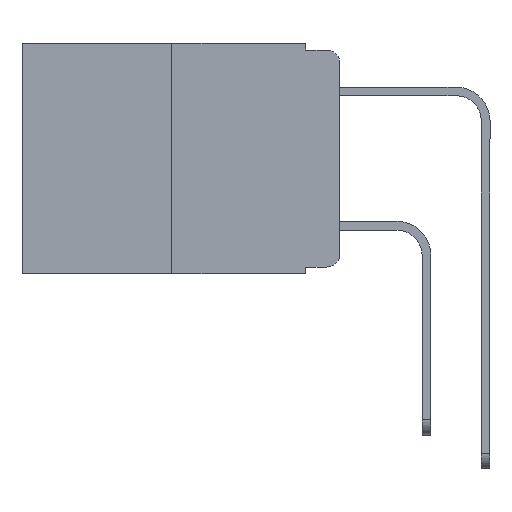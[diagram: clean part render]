
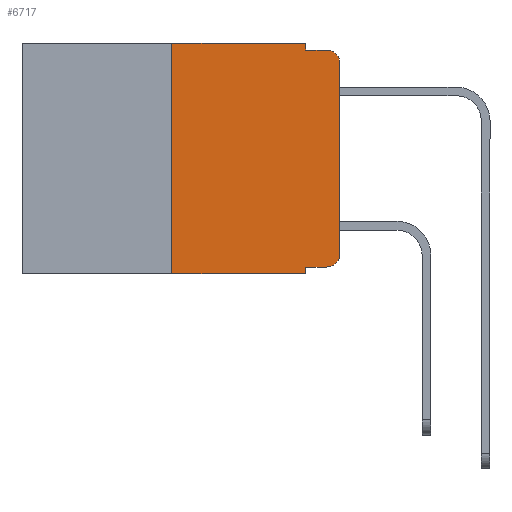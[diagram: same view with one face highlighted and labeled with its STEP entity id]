
A CAD part, left-side view. The second image highlights one B-rep face of the part: STEP entity #6717.
In plain terms, the highlighted planar face has unit normal (-1, 0, 0).
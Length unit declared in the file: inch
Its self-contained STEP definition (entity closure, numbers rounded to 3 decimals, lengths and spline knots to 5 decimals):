
#454 = LINE ( 'NONE', #2485, #11881 ) ;
#506 = DIRECTION ( 'NONE',  ( 0., 0., -1. ) ) ;
#592 = CARTESIAN_POINT ( 'NONE',  ( 0., 0.051, -0.333 ) ) ;
#717 = CIRCLE ( 'NONE', #2835, 0.02 ) ;
#940 = EDGE_CURVE ( 'NONE', #14109, #8351, #7957, .T. ) ;
#1337 = CARTESIAN_POINT ( 'NONE',  ( 0., 0.25, 0. ) ) ;
#1345 = DIRECTION ( 'NONE',  ( 0., 0., 1. ) ) ;
#1373 = VECTOR ( 'NONE', #1345, 39.37008 ) ;
#1735 = VECTOR ( 'NONE', #13034, 39.37008 ) ;
#1844 = EDGE_CURVE ( 'NONE', #14109, #13700, #3982, .T. ) ;
#1927 = VERTEX_POINT ( 'NONE', #11083 ) ;
#2132 = ORIENTED_EDGE ( 'NONE', *, *, #14642, .T. ) ;
#2195 = EDGE_LOOP ( 'NONE', ( #5066, #6469, #6988, #11671, #12996, #7486, #2898, #10226, #9751, #2132 ) ) ;
#2341 = CIRCLE ( 'NONE', #6979, 0.02 ) ;
#2485 = CARTESIAN_POINT ( 'NONE',  ( 0., 0.473, -0.343 ) ) ;
#2699 = EDGE_CURVE ( 'NONE', #11768, #9002, #4660, .T. ) ;
#2835 = AXIS2_PLACEMENT_3D ( 'NONE', #13978, #7622, #506 ) ;
#2898 = ORIENTED_EDGE ( 'NONE', *, *, #3746, .T. ) ;
#3273 = DIRECTION ( 'NONE',  ( -1., 0., 0. ) ) ;
#3292 = CARTESIAN_POINT ( 'NONE',  ( 0., 0.051, -0.01 ) ) ;
#3385 = DIRECTION ( 'NONE',  ( 0., -1., 0. ) ) ;
#3554 = EDGE_CURVE ( 'NONE', #8930, #12982, #8603, .T. ) ;
#3745 = CARTESIAN_POINT ( 'NONE',  ( 0., 0.473, 0. ) ) ;
#3746 = EDGE_CURVE ( 'NONE', #11768, #13700, #454, .T. ) ;
#3982 = LINE ( 'NONE', #14052, #11631 ) ;
#4300 = EDGE_CURVE ( 'NONE', #12982, #7825, #10400, .T. ) ;
#4369 = CARTESIAN_POINT ( 'NONE',  ( 0., 0.051, 0. ) ) ;
#4660 = LINE ( 'NONE', #14540, #1373 ) ;
#5062 = EDGE_CURVE ( 'NONE', #1927, #7825, #2341, .T. ) ;
#5066 = ORIENTED_EDGE ( 'NONE', *, *, #6547, .T. ) ;
#5121 = AXIS2_PLACEMENT_3D ( 'NONE', #10971, #6692, #14125 ) ;
#5256 = CARTESIAN_POINT ( 'NONE',  ( 0., 0.25, -0.343 ) ) ;
#5494 = DIRECTION ( 'NONE',  ( 0., 0., -1. ) ) ;
#5903 = CARTESIAN_POINT ( 'NONE',  ( 0., 0.051, 0. ) ) ;
#6469 = ORIENTED_EDGE ( 'NONE', *, *, #5062, .T. ) ;
#6547 = EDGE_CURVE ( 'NONE', #11022, #1927, #8547, .T. ) ;
#6692 = DIRECTION ( 'NONE',  ( 1., 0., 0. ) ) ;
#6717 = ADVANCED_FACE ( 'NONE', ( #9396 ), #13075, .F. ) ;
#6979 = AXIS2_PLACEMENT_3D ( 'NONE', #9922, #3273, #10957 ) ;
#6988 = ORIENTED_EDGE ( 'NONE', *, *, #4300, .F. ) ;
#7024 = VECTOR ( 'NONE', #7108, 39.37008 ) ;
#7108 = DIRECTION ( 'NONE',  ( 0., -1., 0. ) ) ;
#7441 = CARTESIAN_POINT ( 'NONE',  ( 0., 0., 0. ) ) ;
#7466 = CARTESIAN_POINT ( 'NONE',  ( 0., 0., -0.313 ) ) ;
#7486 = ORIENTED_EDGE ( 'NONE', *, *, #2699, .F. ) ;
#7622 = DIRECTION ( 'NONE',  ( -1., 0., 0. ) ) ;
#7825 = VERTEX_POINT ( 'NONE', #11664 ) ;
#7957 = LINE ( 'NONE', #13167, #12925 ) ;
#8193 = DIRECTION ( 'NONE',  ( 0., -1., 0. ) ) ;
#8351 = VERTEX_POINT ( 'NONE', #10460 ) ;
#8547 = LINE ( 'NONE', #7441, #11015 ) ;
#8603 = LINE ( 'NONE', #4369, #11388 ) ;
#8622 = DIRECTION ( 'NONE',  ( 0., 0., 1. ) ) ;
#8930 = VERTEX_POINT ( 'NONE', #5903 ) ;
#9002 = VERTEX_POINT ( 'NONE', #1337 ) ;
#9396 = FACE_OUTER_BOUND ( 'NONE', #2195, .T. ) ;
#9751 = ORIENTED_EDGE ( 'NONE', *, *, #940, .T. ) ;
#9884 = CARTESIAN_POINT ( 'NONE',  ( 0., 0.051, -0.01 ) ) ;
#9922 = CARTESIAN_POINT ( 'NONE',  ( 0., 0.02, -0.03 ) ) ;
#10226 = ORIENTED_EDGE ( 'NONE', *, *, #1844, .F. ) ;
#10400 = LINE ( 'NONE', #3292, #1735 ) ;
#10460 = CARTESIAN_POINT ( 'NONE',  ( 0., 0.02, -0.333 ) ) ;
#10801 = EDGE_CURVE ( 'NONE', #9002, #8930, #12687, .T. ) ;
#10957 = DIRECTION ( 'NONE',  ( 0., 0., -1. ) ) ;
#10971 = CARTESIAN_POINT ( 'NONE',  ( 0., 0.473, 0. ) ) ;
#11015 = VECTOR ( 'NONE', #8622, 39.37008 ) ;
#11022 = VERTEX_POINT ( 'NONE', #7466 ) ;
#11083 = CARTESIAN_POINT ( 'NONE',  ( 0., 0., -0.03 ) ) ;
#11388 = VECTOR ( 'NONE', #5494, 39.37008 ) ;
#11631 = VECTOR ( 'NONE', #13907, 39.37008 ) ;
#11664 = CARTESIAN_POINT ( 'NONE',  ( 0., 0.02, -0.01 ) ) ;
#11671 = ORIENTED_EDGE ( 'NONE', *, *, #3554, .F. ) ;
#11768 = VERTEX_POINT ( 'NONE', #5256 ) ;
#11881 = VECTOR ( 'NONE', #8193, 39.37008 ) ;
#11898 = CARTESIAN_POINT ( 'NONE',  ( 0., 0.051, -0.343 ) ) ;
#12687 = LINE ( 'NONE', #3745, #7024 ) ;
#12925 = VECTOR ( 'NONE', #3385, 39.37008 ) ;
#12982 = VERTEX_POINT ( 'NONE', #9884 ) ;
#12996 = ORIENTED_EDGE ( 'NONE', *, *, #10801, .F. ) ;
#13034 = DIRECTION ( 'NONE',  ( 0., -1., 0. ) ) ;
#13075 = PLANE ( 'NONE',  #5121 ) ;
#13167 = CARTESIAN_POINT ( 'NONE',  ( 0., 0.051, -0.333 ) ) ;
#13700 = VERTEX_POINT ( 'NONE', #11898 ) ;
#13907 = DIRECTION ( 'NONE',  ( 0., 0., -1. ) ) ;
#13978 = CARTESIAN_POINT ( 'NONE',  ( 0., 0.02, -0.313 ) ) ;
#14052 = CARTESIAN_POINT ( 'NONE',  ( 0., 0.051, 0. ) ) ;
#14109 = VERTEX_POINT ( 'NONE', #592 ) ;
#14125 = DIRECTION ( 'NONE',  ( 0., 0., -1. ) ) ;
#14540 = CARTESIAN_POINT ( 'NONE',  ( 0., 0.25, 0. ) ) ;
#14642 = EDGE_CURVE ( 'NONE', #8351, #11022, #717, .T. ) ;
